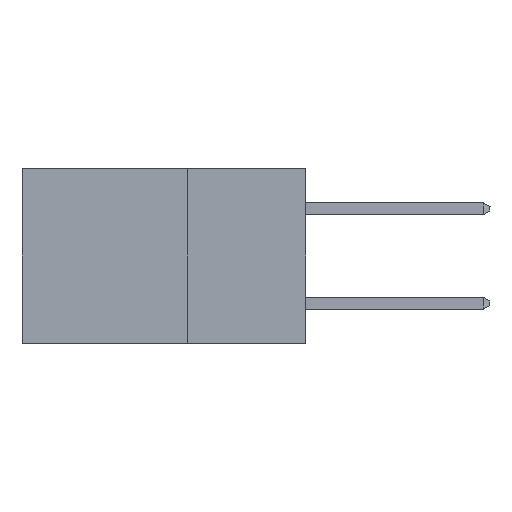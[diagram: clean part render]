
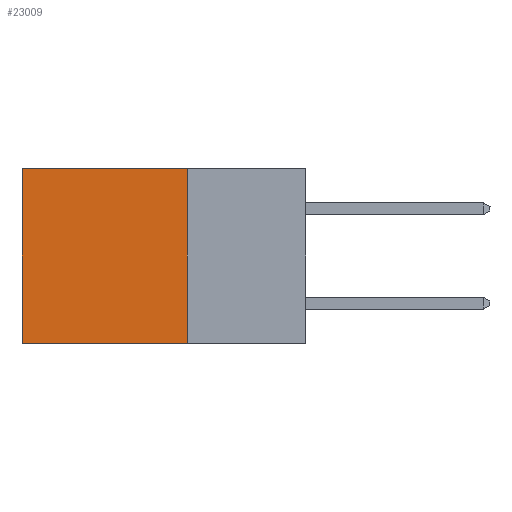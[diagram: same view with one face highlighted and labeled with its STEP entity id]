
A CAD part, left-side view. The second image highlights one B-rep face of the part: STEP entity #23009.
In plain terms, the highlighted planar face has unit normal (-1, 0, 0).
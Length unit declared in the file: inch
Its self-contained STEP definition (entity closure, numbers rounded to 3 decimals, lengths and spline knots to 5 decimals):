
#193 = LINE ( 'NONE', #3654, #23614 ) ;
#376 = CARTESIAN_POINT ( 'NONE',  ( 0.298, 0.25, 0. ) ) ;
#558 = FACE_OUTER_BOUND ( 'NONE', #1196, .T. ) ;
#577 = CARTESIAN_POINT ( 'NONE',  ( 0.298, 0.25, -0.37 ) ) ;
#1196 = EDGE_LOOP ( 'NONE', ( #17536, #19444, #9000, #19877 ) ) ;
#1504 = VERTEX_POINT ( 'NONE', #577 ) ;
#2010 = VERTEX_POINT ( 'NONE', #15652 ) ;
#2207 = VERTEX_POINT ( 'NONE', #3073 ) ;
#2345 = PLANE ( 'NONE',  #23881 ) ;
#3073 = CARTESIAN_POINT ( 'NONE',  ( 0.298, 0.25, 0. ) ) ;
#3215 = LINE ( 'NONE', #23687, #18527 ) ;
#3654 = CARTESIAN_POINT ( 'NONE',  ( 0.298, 0.6, 0. ) ) ;
#5264 = EDGE_CURVE ( 'NONE', #1504, #20580, #3215, .T. ) ;
#5296 = DIRECTION ( 'NONE',  ( 0., 0., -1. ) ) ;
#6447 = DIRECTION ( 'NONE',  ( 0., 1., 0. ) ) ;
#8224 = DIRECTION ( 'NONE',  ( 0., 0., -1. ) ) ;
#8723 = CARTESIAN_POINT ( 'NONE',  ( 0.298, 0.25, 0. ) ) ;
#9000 = ORIENTED_EDGE ( 'NONE', *, *, #14130, .F. ) ;
#14130 = EDGE_CURVE ( 'NONE', #2207, #1504, #14987, .T. ) ;
#14290 = DIRECTION ( 'NONE',  ( 0., 0., -1. ) ) ;
#14388 = EDGE_CURVE ( 'NONE', #2207, #2010, #23733, .T. ) ;
#14987 = LINE ( 'NONE', #21460, #20997 ) ;
#15652 = CARTESIAN_POINT ( 'NONE',  ( 0.298, 0.6, 0. ) ) ;
#17536 = ORIENTED_EDGE ( 'NONE', *, *, #18658, .T. ) ;
#18527 = VECTOR ( 'NONE', #6447, 39.37008 ) ;
#18658 = EDGE_CURVE ( 'NONE', #2010, #20580, #193, .T. ) ;
#19444 = ORIENTED_EDGE ( 'NONE', *, *, #5264, .F. ) ;
#19877 = ORIENTED_EDGE ( 'NONE', *, *, #14388, .T. ) ;
#19892 = CARTESIAN_POINT ( 'NONE',  ( 0.298, 0.6, -0.37 ) ) ;
#20580 = VERTEX_POINT ( 'NONE', #19892 ) ;
#20701 = VECTOR ( 'NONE', #22287, 39.37008 ) ;
#20997 = VECTOR ( 'NONE', #8224, 39.37008 ) ;
#21460 = CARTESIAN_POINT ( 'NONE',  ( 0.298, 0.25, 0. ) ) ;
#21779 = DIRECTION ( 'NONE',  ( 1., 0., 0. ) ) ;
#22287 = DIRECTION ( 'NONE',  ( 0., 1., 0. ) ) ;
#23009 = ADVANCED_FACE ( 'NONE', ( #558 ), #2345, .F. ) ;
#23614 = VECTOR ( 'NONE', #5296, 39.37008 ) ;
#23687 = CARTESIAN_POINT ( 'NONE',  ( 0.298, 0.25, -0.37 ) ) ;
#23733 = LINE ( 'NONE', #8723, #20701 ) ;
#23881 = AXIS2_PLACEMENT_3D ( 'NONE', #376, #21779, #14290 ) ;
